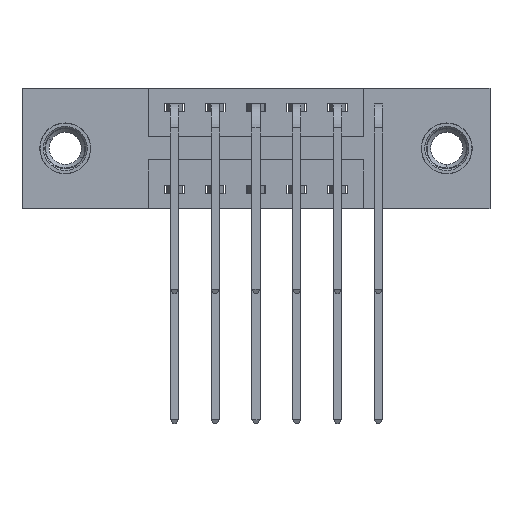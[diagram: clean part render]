
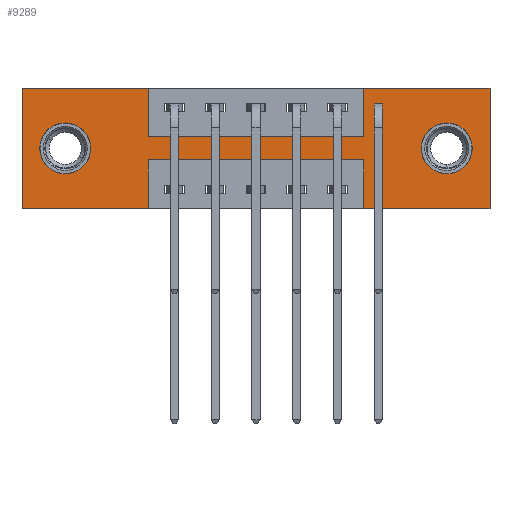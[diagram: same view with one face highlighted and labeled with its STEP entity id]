
A CAD part, front view. The second image highlights one B-rep face of the part: STEP entity #9289.
In plain terms, the highlighted planar face has unit normal (0, -1, 0).
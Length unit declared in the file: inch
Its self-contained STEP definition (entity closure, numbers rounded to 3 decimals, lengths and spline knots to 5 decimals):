
#21 = VERTEX_POINT ( 'NONE', #5849 ) ;
#74 = VECTOR ( 'NONE', #10595, 39.37008 ) ;
#217 = CARTESIAN_POINT ( 'NONE',  ( 0., 0., -0.37 ) ) ;
#327 = EDGE_CURVE ( 'NONE', #650, #21, #3581, .T. ) ;
#362 = CARTESIAN_POINT ( 'NONE',  ( 1.3025, 0., -0.185 ) ) ;
#385 = CIRCLE ( 'NONE', #7138, 0.078 ) ;
#439 = CARTESIAN_POINT ( 'NONE',  ( 0.3875, 0., -0.22 ) ) ;
#561 = ORIENTED_EDGE ( 'NONE', *, *, #4881, .F. ) ;
#593 = DIRECTION ( 'NONE',  ( 0., 0., 1. ) ) ;
#650 = VERTEX_POINT ( 'NONE', #5483 ) ;
#664 = EDGE_CURVE ( 'NONE', #4541, #6343, #9018, .T. ) ;
#778 = CARTESIAN_POINT ( 'NONE',  ( 1.0475, 0., -0.22 ) ) ;
#819 = VECTOR ( 'NONE', #3252, 39.37008 ) ;
#876 = EDGE_CURVE ( 'NONE', #6597, #6444, #6740, .T. ) ;
#971 = ORIENTED_EDGE ( 'NONE', *, *, #876, .F. ) ;
#994 = VERTEX_POINT ( 'NONE', #8679 ) ;
#1158 = DIRECTION ( 'NONE',  ( -1., 0., 0. ) ) ;
#1191 = DIRECTION ( 'NONE',  ( 0., 0., -1. ) ) ;
#1300 = VECTOR ( 'NONE', #7705, 39.37008 ) ;
#1323 = CARTESIAN_POINT ( 'NONE',  ( 1.435, 0., 0. ) ) ;
#1325 = ORIENTED_EDGE ( 'NONE', *, *, #8590, .F. ) ;
#1372 = ORIENTED_EDGE ( 'NONE', *, *, #4929, .F. ) ;
#1379 = ORIENTED_EDGE ( 'NONE', *, *, #6596, .F. ) ;
#1539 = DIRECTION ( 'NONE',  ( 0., 0., -1. ) ) ;
#1626 = ORIENTED_EDGE ( 'NONE', *, *, #8166, .F. ) ;
#1844 = CARTESIAN_POINT ( 'NONE',  ( 0., 0., 0. ) ) ;
#1914 = CARTESIAN_POINT ( 'NONE',  ( 0.1325, 0., -0.185 ) ) ;
#1985 = DIRECTION ( 'NONE',  ( 0., 1., 0. ) ) ;
#2127 = EDGE_CURVE ( 'NONE', #994, #4921, #3433, .T. ) ;
#2282 = EDGE_CURVE ( 'NONE', #10958, #7139, #4038, .T. ) ;
#2311 = DIRECTION ( 'NONE',  ( -1., 0., 0. ) ) ;
#2449 = EDGE_LOOP ( 'NONE', ( #10338, #6161, #2948, #7040, #1379, #3079, #1325, #561, #1626, #1372, #5555, #971 ) ) ;
#2453 = LINE ( 'NONE', #8596, #819 ) ;
#2568 = VERTEX_POINT ( 'NONE', #1844 ) ;
#2730 = VERTEX_POINT ( 'NONE', #7672 ) ;
#2948 = ORIENTED_EDGE ( 'NONE', *, *, #7324, .F. ) ;
#2956 = DIRECTION ( 'NONE',  ( 0., 0., -1. ) ) ;
#3079 = ORIENTED_EDGE ( 'NONE', *, *, #2282, .F. ) ;
#3252 = DIRECTION ( 'NONE',  ( 0., 0., -1. ) ) ;
#3281 = CARTESIAN_POINT ( 'NONE',  ( 0., 0., 0. ) ) ;
#3395 = AXIS2_PLACEMENT_3D ( 'NONE', #362, #1985, #1539 ) ;
#3433 = CIRCLE ( 'NONE', #3983, 0.078 ) ;
#3451 = DIRECTION ( 'NONE',  ( 0., 0., 1. ) ) ;
#3504 = LINE ( 'NONE', #10448, #8844 ) ;
#3565 = EDGE_CURVE ( 'NONE', #4902, #9319, #10236, .T. ) ;
#3581 = CIRCLE ( 'NONE', #3395, 0.078 ) ;
#3610 = EDGE_CURVE ( 'NONE', #4921, #994, #385, .T. ) ;
#3627 = DIRECTION ( 'NONE',  ( 0., 1., 0. ) ) ;
#3676 = DIRECTION ( 'NONE',  ( 0., -1., 0. ) ) ;
#3794 = DIRECTION ( 'NONE',  ( 0., 1., 0. ) ) ;
#3896 = CIRCLE ( 'NONE', #8310, 0.078 ) ;
#3958 = VECTOR ( 'NONE', #11271, 39.37008 ) ;
#3983 = AXIS2_PLACEMENT_3D ( 'NONE', #1914, #3794, #8851 ) ;
#4038 = LINE ( 'NONE', #3281, #4912 ) ;
#4052 = CARTESIAN_POINT ( 'NONE',  ( 1.0475, 0., -0.37 ) ) ;
#4541 = VERTEX_POINT ( 'NONE', #778 ) ;
#4554 = PLANE ( 'NONE',  #11028 ) ;
#4853 = CARTESIAN_POINT ( 'NONE',  ( 1.435, 0., -0.37 ) ) ;
#4881 = EDGE_CURVE ( 'NONE', #5337, #8131, #10289, .T. ) ;
#4901 = DIRECTION ( 'NONE',  ( 1., 0., 0. ) ) ;
#4902 = VERTEX_POINT ( 'NONE', #4853 ) ;
#4912 = VECTOR ( 'NONE', #4901, 39.37008 ) ;
#4921 = VERTEX_POINT ( 'NONE', #11198 ) ;
#4929 = EDGE_CURVE ( 'NONE', #2568, #2730, #11140, .T. ) ;
#5337 = VERTEX_POINT ( 'NONE', #10042 ) ;
#5483 = CARTESIAN_POINT ( 'NONE',  ( 1.3025, 0., -0.107 ) ) ;
#5555 = ORIENTED_EDGE ( 'NONE', *, *, #10735, .F. ) ;
#5696 = DIRECTION ( 'NONE',  ( -1., 0., 0. ) ) ;
#5833 = CARTESIAN_POINT ( 'NONE',  ( 1.0475, 0., 0. ) ) ;
#5849 = CARTESIAN_POINT ( 'NONE',  ( 1.3025, 0., -0.263 ) ) ;
#5909 = CARTESIAN_POINT ( 'NONE',  ( 0., 0., -0.37 ) ) ;
#5930 = DIRECTION ( 'NONE',  ( 0., 0., 1. ) ) ;
#6161 = ORIENTED_EDGE ( 'NONE', *, *, #664, .F. ) ;
#6266 = FACE_BOUND ( 'NONE', #10520, .T. ) ;
#6343 = VERTEX_POINT ( 'NONE', #439 ) ;
#6444 = VERTEX_POINT ( 'NONE', #5909 ) ;
#6536 = ORIENTED_EDGE ( 'NONE', *, *, #9196, .T. ) ;
#6560 = DIRECTION ( 'NONE',  ( 0., 1., 0. ) ) ;
#6596 = EDGE_CURVE ( 'NONE', #7139, #4902, #7164, .T. ) ;
#6597 = VERTEX_POINT ( 'NONE', #7978 ) ;
#6702 = VECTOR ( 'NONE', #2311, 39.37008 ) ;
#6740 = LINE ( 'NONE', #10240, #6702 ) ;
#6797 = DIRECTION ( 'NONE',  ( 1., 0., 0. ) ) ;
#6819 = CARTESIAN_POINT ( 'NONE',  ( 1.0475, 0., -0.15 ) ) ;
#6925 = ORIENTED_EDGE ( 'NONE', *, *, #2127, .T. ) ;
#6973 = DIRECTION ( 'NONE',  ( 0., 0., -1. ) ) ;
#7040 = ORIENTED_EDGE ( 'NONE', *, *, #3565, .F. ) ;
#7138 = AXIS2_PLACEMENT_3D ( 'NONE', #8571, #6560, #5930 ) ;
#7139 = VERTEX_POINT ( 'NONE', #1323 ) ;
#7164 = LINE ( 'NONE', #9676, #74 ) ;
#7212 = EDGE_LOOP ( 'NONE', ( #9388, #6925 ) ) ;
#7316 = VECTOR ( 'NONE', #5696, 39.37008 ) ;
#7324 = EDGE_CURVE ( 'NONE', #9319, #4541, #11149, .T. ) ;
#7590 = CARTESIAN_POINT ( 'NONE',  ( 0.3875, 0., -0.15 ) ) ;
#7672 = CARTESIAN_POINT ( 'NONE',  ( 0.3875, 0., 0. ) ) ;
#7685 = VECTOR ( 'NONE', #6797, 39.37008 ) ;
#7705 = DIRECTION ( 'NONE',  ( 1., 0., 0. ) ) ;
#7723 = VECTOR ( 'NONE', #593, 39.37008 ) ;
#7917 = ORIENTED_EDGE ( 'NONE', *, *, #327, .T. ) ;
#7931 = VECTOR ( 'NONE', #2956, 39.37008 ) ;
#7978 = CARTESIAN_POINT ( 'NONE',  ( 0.3875, 0., -0.37 ) ) ;
#8015 = EDGE_CURVE ( 'NONE', #6343, #6597, #8491, .T. ) ;
#8089 = CARTESIAN_POINT ( 'NONE',  ( 1.0475, 0., 0. ) ) ;
#8131 = VERTEX_POINT ( 'NONE', #6819 ) ;
#8166 = EDGE_CURVE ( 'NONE', #2730, #5337, #2453, .T. ) ;
#8310 = AXIS2_PLACEMENT_3D ( 'NONE', #8729, #3627, #6973 ) ;
#8471 = LINE ( 'NONE', #5833, #3958 ) ;
#8491 = LINE ( 'NONE', #9097, #7931 ) ;
#8571 = CARTESIAN_POINT ( 'NONE',  ( 0.1325, 0., -0.185 ) ) ;
#8590 = EDGE_CURVE ( 'NONE', #8131, #10958, #8471, .T. ) ;
#8596 = CARTESIAN_POINT ( 'NONE',  ( 0.3875, 0., 0. ) ) ;
#8679 = CARTESIAN_POINT ( 'NONE',  ( 0.1325, 0., -0.263 ) ) ;
#8729 = CARTESIAN_POINT ( 'NONE',  ( 1.3025, 0., -0.185 ) ) ;
#8844 = VECTOR ( 'NONE', #3451, 39.37008 ) ;
#8851 = DIRECTION ( 'NONE',  ( 0., 0., 1. ) ) ;
#8896 = FACE_OUTER_BOUND ( 'NONE', #2449, .T. ) ;
#9002 = CARTESIAN_POINT ( 'NONE',  ( 1.0475, 0., -0.37 ) ) ;
#9018 = LINE ( 'NONE', #10581, #10897 ) ;
#9097 = CARTESIAN_POINT ( 'NONE',  ( 0.3875, 0., -0.37 ) ) ;
#9196 = EDGE_CURVE ( 'NONE', #21, #650, #3896, .T. ) ;
#9289 = ADVANCED_FACE ( 'NONE', ( #6266, #9751, #8896 ), #4554, .T. ) ;
#9319 = VERTEX_POINT ( 'NONE', #9002 ) ;
#9360 = CARTESIAN_POINT ( 'NONE',  ( 0., 0., 0. ) ) ;
#9388 = ORIENTED_EDGE ( 'NONE', *, *, #3610, .T. ) ;
#9676 = CARTESIAN_POINT ( 'NONE',  ( 1.435, 0., 0. ) ) ;
#9751 = FACE_BOUND ( 'NONE', #7212, .T. ) ;
#10042 = CARTESIAN_POINT ( 'NONE',  ( 0.3875, 0., -0.15 ) ) ;
#10236 = LINE ( 'NONE', #10287, #7316 ) ;
#10240 = CARTESIAN_POINT ( 'NONE',  ( 0., 0., -0.37 ) ) ;
#10287 = CARTESIAN_POINT ( 'NONE',  ( 0., 0., -0.37 ) ) ;
#10289 = LINE ( 'NONE', #7590, #1300 ) ;
#10338 = ORIENTED_EDGE ( 'NONE', *, *, #8015, .F. ) ;
#10448 = CARTESIAN_POINT ( 'NONE',  ( 0., 0., 0. ) ) ;
#10520 = EDGE_LOOP ( 'NONE', ( #7917, #6536 ) ) ;
#10581 = CARTESIAN_POINT ( 'NONE',  ( 0.3875, 0., -0.22 ) ) ;
#10595 = DIRECTION ( 'NONE',  ( 0., 0., -1. ) ) ;
#10735 = EDGE_CURVE ( 'NONE', #6444, #2568, #3504, .T. ) ;
#10897 = VECTOR ( 'NONE', #1158, 39.37008 ) ;
#10958 = VERTEX_POINT ( 'NONE', #8089 ) ;
#11028 = AXIS2_PLACEMENT_3D ( 'NONE', #217, #3676, #1191 ) ;
#11140 = LINE ( 'NONE', #9360, #7685 ) ;
#11149 = LINE ( 'NONE', #4052, #7723 ) ;
#11198 = CARTESIAN_POINT ( 'NONE',  ( 0.1325, 0., -0.107 ) ) ;
#11271 = DIRECTION ( 'NONE',  ( 0., 0., 1. ) ) ;
